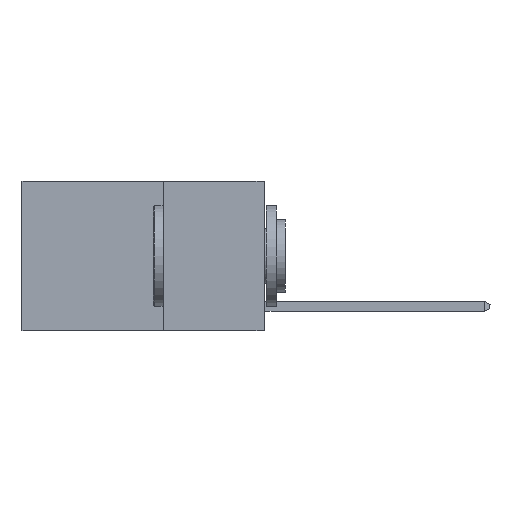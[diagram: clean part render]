
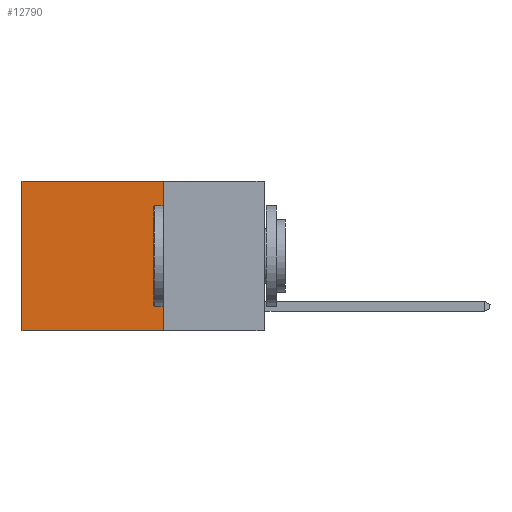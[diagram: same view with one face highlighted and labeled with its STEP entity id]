
A CAD part, left-side view. The second image highlights one B-rep face of the part: STEP entity #12790.
In plain terms, the highlighted planar face has unit normal (-1, 0, 0).
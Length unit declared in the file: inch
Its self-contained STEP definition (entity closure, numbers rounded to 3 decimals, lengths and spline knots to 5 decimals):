
#945 = CARTESIAN_POINT ( 'NONE',  ( 0.2625, 0.6, -0.37 ) ) ;
#1255 = CARTESIAN_POINT ( 'NONE',  ( 0.2625, 0.25, 0. ) ) ;
#1712 = AXIS2_PLACEMENT_3D ( 'NONE', #12604, #5889, #12478 ) ;
#2572 = CARTESIAN_POINT ( 'NONE',  ( 0.2625, 0.6, 0. ) ) ;
#3055 = VERTEX_POINT ( 'NONE', #2572 ) ;
#4240 = VECTOR ( 'NONE', #10883, 39.37008 ) ;
#5044 = LINE ( 'NONE', #9886, #11674 ) ;
#5423 = VERTEX_POINT ( 'NONE', #15024 ) ;
#5776 = EDGE_CURVE ( 'NONE', #3055, #10387, #5044, .T. ) ;
#5885 = ORIENTED_EDGE ( 'NONE', *, *, #8988, .F. ) ;
#5889 = DIRECTION ( 'NONE',  ( 1., 0., 0. ) ) ;
#6004 = LINE ( 'NONE', #6847, #9332 ) ;
#6725 = EDGE_CURVE ( 'NONE', #15038, #5423, #10231, .T. ) ;
#6847 = CARTESIAN_POINT ( 'NONE',  ( 0.2625, 0.25, 0. ) ) ;
#8724 = LINE ( 'NONE', #14994, #9148 ) ;
#8726 = DIRECTION ( 'NONE',  ( 0., 0., -1. ) ) ;
#8755 = ORIENTED_EDGE ( 'NONE', *, *, #5776, .T. ) ;
#8988 = EDGE_CURVE ( 'NONE', #5423, #10387, #8724, .T. ) ;
#9148 = VECTOR ( 'NONE', #9883, 39.37008 ) ;
#9332 = VECTOR ( 'NONE', #10987, 39.37008 ) ;
#9414 = EDGE_CURVE ( 'NONE', #15038, #3055, #6004, .T. ) ;
#9725 = CARTESIAN_POINT ( 'NONE',  ( 0.2625, 0.25, 0. ) ) ;
#9883 = DIRECTION ( 'NONE',  ( 0., 1., 0. ) ) ;
#9886 = CARTESIAN_POINT ( 'NONE',  ( 0.2625, 0.6, 0. ) ) ;
#10032 = ORIENTED_EDGE ( 'NONE', *, *, #6725, .F. ) ;
#10231 = LINE ( 'NONE', #9725, #4240 ) ;
#10387 = VERTEX_POINT ( 'NONE', #945 ) ;
#10883 = DIRECTION ( 'NONE',  ( 0., 0., -1. ) ) ;
#10987 = DIRECTION ( 'NONE',  ( 0., 1., 0. ) ) ;
#11092 = ORIENTED_EDGE ( 'NONE', *, *, #9414, .T. ) ;
#11298 = PLANE ( 'NONE',  #1712 ) ;
#11674 = VECTOR ( 'NONE', #8726, 39.37008 ) ;
#12478 = DIRECTION ( 'NONE',  ( 0., 0., -1. ) ) ;
#12604 = CARTESIAN_POINT ( 'NONE',  ( 0.2625, 0.25, 0. ) ) ;
#12790 = ADVANCED_FACE ( 'NONE', ( #13180 ), #11298, .F. ) ;
#13180 = FACE_OUTER_BOUND ( 'NONE', #13918, .T. ) ;
#13918 = EDGE_LOOP ( 'NONE', ( #8755, #5885, #10032, #11092 ) ) ;
#14994 = CARTESIAN_POINT ( 'NONE',  ( 0.2625, 0.25, -0.37 ) ) ;
#15024 = CARTESIAN_POINT ( 'NONE',  ( 0.2625, 0.25, -0.37 ) ) ;
#15038 = VERTEX_POINT ( 'NONE', #1255 ) ;
